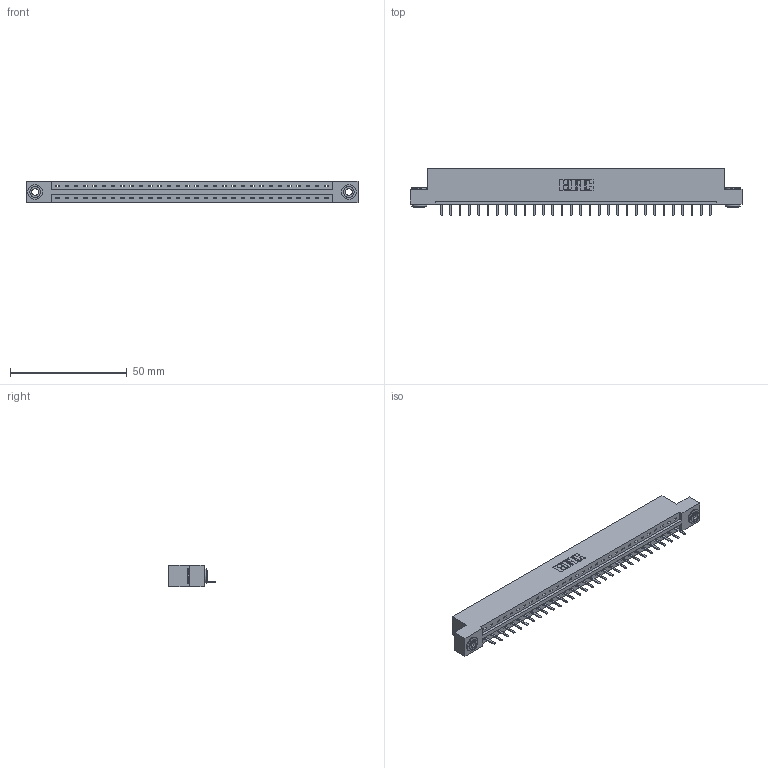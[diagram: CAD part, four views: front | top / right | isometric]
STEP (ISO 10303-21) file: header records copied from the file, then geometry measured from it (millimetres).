
FILE_DESCRIPTION (( 'STEP AP203' ), '1' );
FILE_NAME ('387-030-520-103.STEP', '2019-10-03T17:41:34', ( '' ), ( '' ), 'SwSTEP 2.0', 'SolidWorks 2016', '' );
FILE_SCHEMA (( 'CONFIG_CONTROL_DESIGN' ));
Length unit declared in the file: inch
Products named in the file (4): 337 Part_Flush Mounting Lugs - 0.156 Dia-TH; 345-250-002_345-250-002-102; 345-292-001_345-293-120; 387-030-520-103
Assembly tree (33 placements, depth 2):
  387-030-520-103
    337 Part_Flush Mounting Lugs - 0.156 Dia-TH
    345-292-001_345-293-120  x30
    345-250-002_345-250-002-102  x2
Bounding box: 141.88 x 20.02 x 9.4 mm (x, y, z)
Volume: 14529.4 mm3; surface area: 14869.5 mm2
Topology: 33 solids, 33 shells, 2132 faces, 6267 edges, 4094 vertices
Faces by surface type: plane 1520, cylinder 604, cone 8
Entity records: 24616 total; most frequent: CARTESIAN_POINT 4275, ORIENTED_EDGE 4222, DIRECTION 3645, EDGE_CURVE 2111, VECTOR 1955, LINE 1955, VERTEX_POINT 1402, AXIS2_PLACEMENT_3D 845
